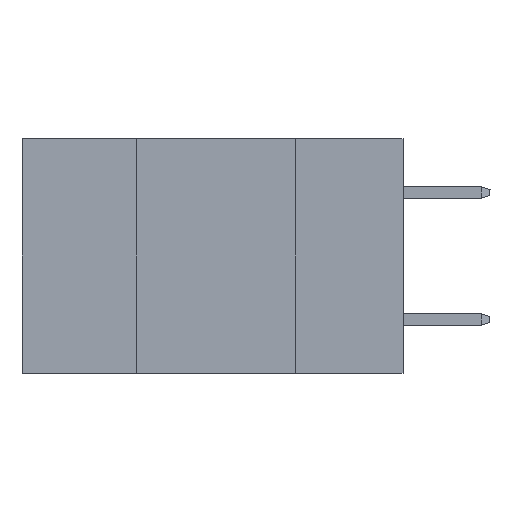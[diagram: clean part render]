
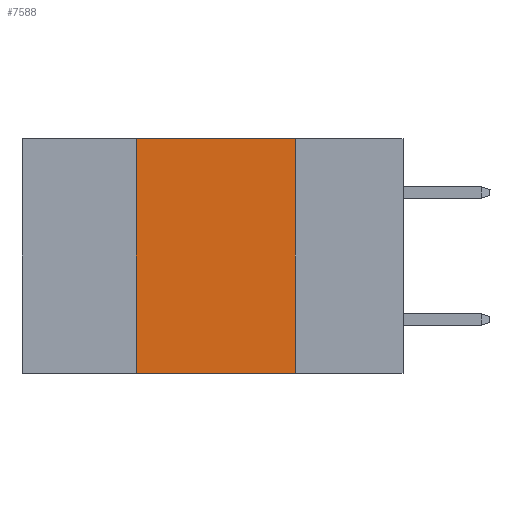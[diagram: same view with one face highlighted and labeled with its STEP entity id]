
A CAD part, left-side view. The second image highlights one B-rep face of the part: STEP entity #7588.
In plain terms, the highlighted planar face has unit normal (-1, 0, 0).
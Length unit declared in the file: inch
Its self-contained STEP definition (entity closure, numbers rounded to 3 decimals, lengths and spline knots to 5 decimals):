
#321 = DIRECTION ( 'NONE',  ( 1., 0., 0. ) ) ;
#496 = VERTEX_POINT ( 'NONE', #12420 ) ;
#807 = CARTESIAN_POINT ( 'NONE',  ( 0., 0.42, 0. ) ) ;
#3369 = VECTOR ( 'NONE', #19854, 39.37008 ) ;
#4582 = VERTEX_POINT ( 'NONE', #807 ) ;
#4831 = EDGE_CURVE ( 'NONE', #4582, #35559, #20062, .T. ) ;
#6045 = EDGE_CURVE ( 'NONE', #24721, #496, #17812, .T. ) ;
#7244 = ORIENTED_EDGE ( 'NONE', *, *, #6045, .T. ) ;
#7588 = ADVANCED_FACE ( 'NONE', ( #28751 ), #26017, .F. ) ;
#8101 = CARTESIAN_POINT ( 'NONE',  ( 0., 0.17, 0. ) ) ;
#10066 = EDGE_CURVE ( 'NONE', #35559, #496, #36274, .T. ) ;
#10378 = CARTESIAN_POINT ( 'NONE',  ( 0., 0.6, 0. ) ) ;
#11446 = ORIENTED_EDGE ( 'NONE', *, *, #10066, .F. ) ;
#12420 = CARTESIAN_POINT ( 'NONE',  ( 0., 0.17, -0.37 ) ) ;
#14806 = EDGE_LOOP ( 'NONE', ( #11446, #36758, #37463, #7244 ) ) ;
#14930 = DIRECTION ( 'NONE',  ( 0., 0., 1. ) ) ;
#17812 = LINE ( 'NONE', #36735, #19300 ) ;
#19300 = VECTOR ( 'NONE', #30652, 39.37008 ) ;
#19854 = DIRECTION ( 'NONE',  ( 0., -1., 0. ) ) ;
#20062 = LINE ( 'NONE', #10378, #3369 ) ;
#20486 = VECTOR ( 'NONE', #36480, 39.37008 ) ;
#23275 = DIRECTION ( 'NONE',  ( 0., 0., -1. ) ) ;
#23770 = LINE ( 'NONE', #30702, #41303 ) ;
#24721 = VERTEX_POINT ( 'NONE', #33488 ) ;
#25836 = CARTESIAN_POINT ( 'NONE',  ( 0., 0.17, 0. ) ) ;
#26017 = PLANE ( 'NONE',  #37294 ) ;
#28751 = FACE_OUTER_BOUND ( 'NONE', #14806, .T. ) ;
#30652 = DIRECTION ( 'NONE',  ( 0., -1., 0. ) ) ;
#30702 = CARTESIAN_POINT ( 'NONE',  ( 0., 0.42, 0. ) ) ;
#32325 = CARTESIAN_POINT ( 'NONE',  ( 0., 0.6, 0. ) ) ;
#33488 = CARTESIAN_POINT ( 'NONE',  ( 0., 0.42, -0.37 ) ) ;
#35559 = VERTEX_POINT ( 'NONE', #25836 ) ;
#36274 = LINE ( 'NONE', #8101, #20486 ) ;
#36480 = DIRECTION ( 'NONE',  ( 0., 0., -1. ) ) ;
#36735 = CARTESIAN_POINT ( 'NONE',  ( 0., 0.6, -0.37 ) ) ;
#36758 = ORIENTED_EDGE ( 'NONE', *, *, #4831, .F. ) ;
#37294 = AXIS2_PLACEMENT_3D ( 'NONE', #32325, #321, #23275 ) ;
#37463 = ORIENTED_EDGE ( 'NONE', *, *, #37867, .F. ) ;
#37867 = EDGE_CURVE ( 'NONE', #24721, #4582, #23770, .T. ) ;
#41303 = VECTOR ( 'NONE', #14930, 39.37008 ) ;
